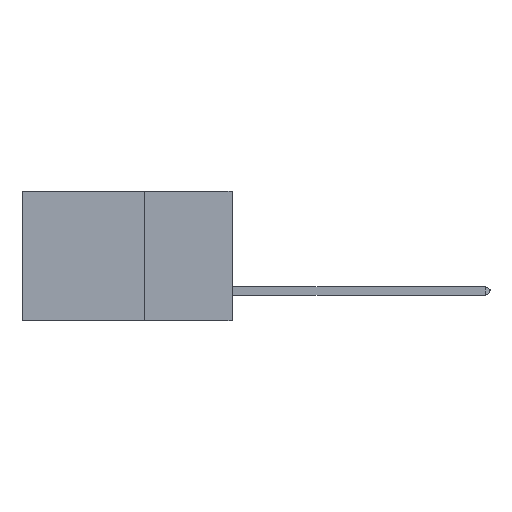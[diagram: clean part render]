
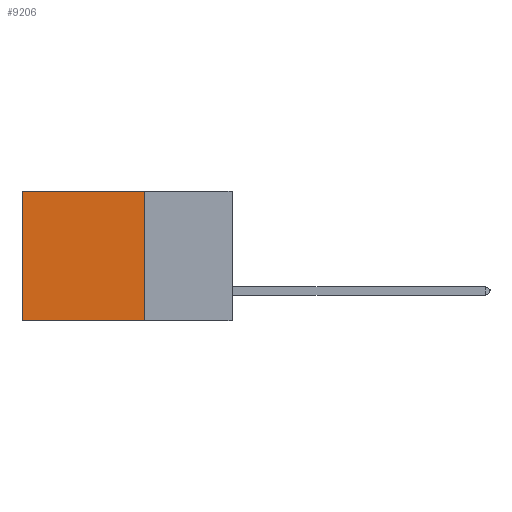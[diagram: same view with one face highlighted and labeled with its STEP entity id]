
A CAD part, left-side view. The second image highlights one B-rep face of the part: STEP entity #9206.
In plain terms, the highlighted planar face has unit normal (-1, 0, 0).
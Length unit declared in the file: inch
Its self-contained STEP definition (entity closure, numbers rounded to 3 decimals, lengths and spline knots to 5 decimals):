
#184 = DIRECTION ( 'NONE',  ( 0., 0., -1. ) ) ;
#767 = DIRECTION ( 'NONE',  ( 0., 0., -1. ) ) ;
#1131 = EDGE_CURVE ( 'NONE', #15086, #25420, #2751, .T. ) ;
#1907 = EDGE_CURVE ( 'NONE', #15086, #13161, #20067, .T. ) ;
#2523 = DIRECTION ( 'NONE',  ( 0., 0., -1. ) ) ;
#2751 = LINE ( 'NONE', #10608, #10035 ) ;
#3938 = CARTESIAN_POINT ( 'NONE',  ( 0.2875, 0.6, -0.37 ) ) ;
#4886 = DIRECTION ( 'NONE',  ( 0., 1., 0. ) ) ;
#4894 = DIRECTION ( 'NONE',  ( 1., 0., 0. ) ) ;
#5017 = CARTESIAN_POINT ( 'NONE',  ( 0.2875, 0.25, -0.37 ) ) ;
#6224 = CARTESIAN_POINT ( 'NONE',  ( 0.2875, 0.25, -0.37 ) ) ;
#6596 = CARTESIAN_POINT ( 'NONE',  ( 0.2875, 0.6, 0. ) ) ;
#6763 = LINE ( 'NONE', #6224, #15604 ) ;
#8518 = CARTESIAN_POINT ( 'NONE',  ( 0.2875, 0.25, 0. ) ) ;
#8840 = ORIENTED_EDGE ( 'NONE', *, *, #1907, .F. ) ;
#8889 = CARTESIAN_POINT ( 'NONE',  ( 0.2875, 0.6, 0. ) ) ;
#9206 = ADVANCED_FACE ( 'NONE', ( #21001 ), #11475, .F. ) ;
#9536 = EDGE_LOOP ( 'NONE', ( #17335, #11194, #8840, #25524 ) ) ;
#10035 = VECTOR ( 'NONE', #4886, 39.37008 ) ;
#10608 = CARTESIAN_POINT ( 'NONE',  ( 0.2875, 0.25, 0. ) ) ;
#11194 = ORIENTED_EDGE ( 'NONE', *, *, #14062, .F. ) ;
#11442 = CARTESIAN_POINT ( 'NONE',  ( 0.2875, 0.25, 0. ) ) ;
#11475 = PLANE ( 'NONE',  #15953 ) ;
#13161 = VERTEX_POINT ( 'NONE', #5017 ) ;
#13366 = VERTEX_POINT ( 'NONE', #3938 ) ;
#14062 = EDGE_CURVE ( 'NONE', #13161, #13366, #6763, .T. ) ;
#14659 = EDGE_CURVE ( 'NONE', #25420, #13366, #23159, .T. ) ;
#14710 = VECTOR ( 'NONE', #184, 39.37008 ) ;
#15086 = VERTEX_POINT ( 'NONE', #11442 ) ;
#15604 = VECTOR ( 'NONE', #20951, 39.37008 ) ;
#15953 = AXIS2_PLACEMENT_3D ( 'NONE', #8518, #4894, #2523 ) ;
#17335 = ORIENTED_EDGE ( 'NONE', *, *, #14659, .T. ) ;
#19823 = CARTESIAN_POINT ( 'NONE',  ( 0.2875, 0.25, 0. ) ) ;
#20067 = LINE ( 'NONE', #19823, #14710 ) ;
#20951 = DIRECTION ( 'NONE',  ( 0., 1., 0. ) ) ;
#21001 = FACE_OUTER_BOUND ( 'NONE', #9536, .T. ) ;
#23159 = LINE ( 'NONE', #8889, #25270 ) ;
#25270 = VECTOR ( 'NONE', #767, 39.37008 ) ;
#25420 = VERTEX_POINT ( 'NONE', #6596 ) ;
#25524 = ORIENTED_EDGE ( 'NONE', *, *, #1131, .T. ) ;
